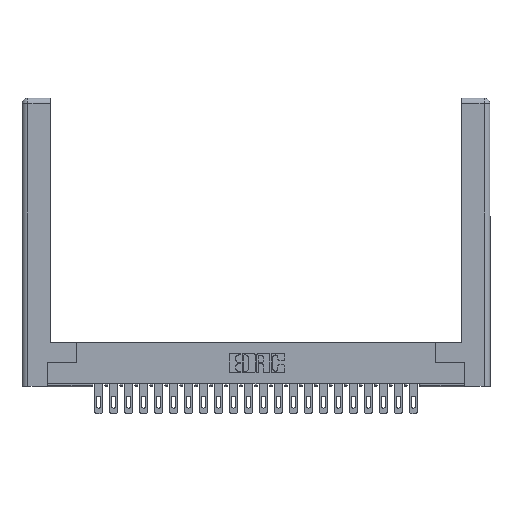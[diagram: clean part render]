
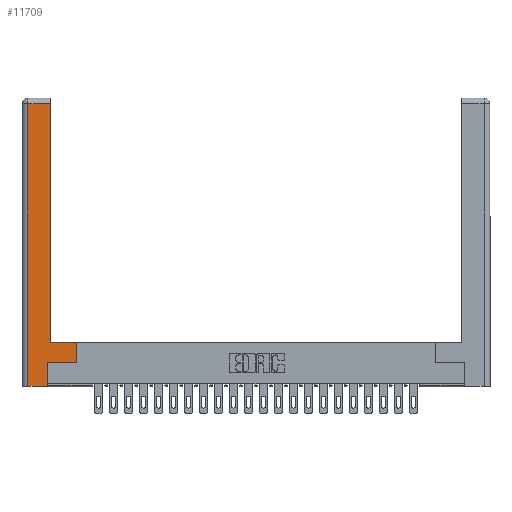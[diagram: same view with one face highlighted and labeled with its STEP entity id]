
A CAD part, top view. The second image highlights one B-rep face of the part: STEP entity #11709.
In plain terms, the highlighted planar face has unit normal (0, 0, 1).
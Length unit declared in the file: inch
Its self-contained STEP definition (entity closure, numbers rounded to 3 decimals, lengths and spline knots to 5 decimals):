
#30 = VECTOR ( 'NONE', #4873, 39.37008 ) ;
#86 = EDGE_CURVE ( 'NONE', #2580, #2665, #5890, .T. ) ;
#1006 = CARTESIAN_POINT ( 'NONE',  ( 0.0615, 2.94, 0. ) ) ;
#1077 = EDGE_CURVE ( 'NONE', #2665, #10648, #22975, .T. ) ;
#1743 = ORIENTED_EDGE ( 'NONE', *, *, #7577, .T. ) ;
#2580 = VERTEX_POINT ( 'NONE', #10593 ) ;
#2665 = VERTEX_POINT ( 'NONE', #12175 ) ;
#3704 = EDGE_LOOP ( 'NONE', ( #20453, #13679, #1743, #4742, #23100, #13297, #11654, #8114 ) ) ;
#4268 = VERTEX_POINT ( 'NONE', #21868 ) ;
#4742 = ORIENTED_EDGE ( 'NONE', *, *, #86, .T. ) ;
#4873 = DIRECTION ( 'NONE',  ( 0., 1., 0. ) ) ;
#4985 = LINE ( 'NONE', #13018, #13797 ) ;
#5576 = CARTESIAN_POINT ( 'NONE',  ( 0.565, 0.245, 0. ) ) ;
#5744 = CARTESIAN_POINT ( 'NONE',  ( 0.265, 0., 0. ) ) ;
#5890 = LINE ( 'NONE', #5744, #17512 ) ;
#6529 = DIRECTION ( 'NONE',  ( 0., 1., 0. ) ) ;
#7114 = DIRECTION ( 'NONE',  ( -1., 0., 0. ) ) ;
#7507 = VERTEX_POINT ( 'NONE', #16440 ) ;
#7577 = EDGE_CURVE ( 'NONE', #19471, #2580, #22825, .T. ) ;
#7915 = DIRECTION ( 'NONE',  ( 0., 0., -1. ) ) ;
#8114 = ORIENTED_EDGE ( 'NONE', *, *, #12169, .T. ) ;
#8278 = VECTOR ( 'NONE', #24922, 39.37008 ) ;
#8797 = EDGE_CURVE ( 'NONE', #4268, #19471, #19155, .T. ) ;
#9209 = CARTESIAN_POINT ( 'NONE',  ( 0.0615, 2.94, 0. ) ) ;
#9589 = CARTESIAN_POINT ( 'NONE',  ( 0.295, 0.45, 0. ) ) ;
#9928 = LINE ( 'NONE', #16227, #25656 ) ;
#9991 = VERTEX_POINT ( 'NONE', #5576 ) ;
#10003 = CARTESIAN_POINT ( 'NONE',  ( 0.265, 0.245, 0. ) ) ;
#10066 = AXIS2_PLACEMENT_3D ( 'NONE', #21660, #7915, #23891 ) ;
#10488 = CARTESIAN_POINT ( 'NONE',  ( 0.565, 0.45, 0. ) ) ;
#10593 = CARTESIAN_POINT ( 'NONE',  ( 0.0615, 0., 0. ) ) ;
#10648 = VERTEX_POINT ( 'NONE', #10003 ) ;
#11654 = ORIENTED_EDGE ( 'NONE', *, *, #23310, .T. ) ;
#11709 = ADVANCED_FACE ( 'NONE', ( #17361 ), #17755, .F. ) ;
#12169 = EDGE_CURVE ( 'NONE', #21334, #7507, #21245, .T. ) ;
#12175 = CARTESIAN_POINT ( 'NONE',  ( 0.265, 0., 0. ) ) ;
#13018 = CARTESIAN_POINT ( 'NONE',  ( 0.295, 3., 0. ) ) ;
#13297 = ORIENTED_EDGE ( 'NONE', *, *, #24865, .T. ) ;
#13560 = EDGE_CURVE ( 'NONE', #7507, #4268, #4985, .T. ) ;
#13679 = ORIENTED_EDGE ( 'NONE', *, *, #8797, .T. ) ;
#13797 = VECTOR ( 'NONE', #20851, 39.37008 ) ;
#16227 = CARTESIAN_POINT ( 'NONE',  ( 0.565, 0.245, 0. ) ) ;
#16386 = LINE ( 'NONE', #10488, #22650 ) ;
#16440 = CARTESIAN_POINT ( 'NONE',  ( 0.295, 0.45, 0. ) ) ;
#17361 = FACE_OUTER_BOUND ( 'NONE', #3704, .T. ) ;
#17438 = VECTOR ( 'NONE', #17587, 39.37008 ) ;
#17512 = VECTOR ( 'NONE', #17822, 39.37008 ) ;
#17587 = DIRECTION ( 'NONE',  ( -1., 0., 0. ) ) ;
#17755 = PLANE ( 'NONE',  #10066 ) ;
#17822 = DIRECTION ( 'NONE',  ( 1., 0., 0. ) ) ;
#18903 = CARTESIAN_POINT ( 'NONE',  ( 0.0615, 0., 0. ) ) ;
#19155 = LINE ( 'NONE', #9209, #20884 ) ;
#19471 = VERTEX_POINT ( 'NONE', #1006 ) ;
#20453 = ORIENTED_EDGE ( 'NONE', *, *, #13560, .T. ) ;
#20851 = DIRECTION ( 'NONE',  ( 0., 1., 0. ) ) ;
#20883 = CARTESIAN_POINT ( 'NONE',  ( 0.265, 0.245, 0. ) ) ;
#20884 = VECTOR ( 'NONE', #7114, 39.37008 ) ;
#21245 = LINE ( 'NONE', #9589, #17438 ) ;
#21334 = VERTEX_POINT ( 'NONE', #22334 ) ;
#21660 = CARTESIAN_POINT ( 'NONE',  ( 0., 0., 0. ) ) ;
#21868 = CARTESIAN_POINT ( 'NONE',  ( 0.295, 2.94, 0. ) ) ;
#22334 = CARTESIAN_POINT ( 'NONE',  ( 0.565, 0.45, 0. ) ) ;
#22650 = VECTOR ( 'NONE', #6529, 39.37008 ) ;
#22825 = LINE ( 'NONE', #18903, #8278 ) ;
#22975 = LINE ( 'NONE', #20883, #30 ) ;
#23100 = ORIENTED_EDGE ( 'NONE', *, *, #1077, .T. ) ;
#23310 = EDGE_CURVE ( 'NONE', #9991, #21334, #16386, .T. ) ;
#23891 = DIRECTION ( 'NONE',  ( -1., 0., 0. ) ) ;
#23951 = DIRECTION ( 'NONE',  ( 1., 0., 0. ) ) ;
#24865 = EDGE_CURVE ( 'NONE', #10648, #9991, #9928, .T. ) ;
#24922 = DIRECTION ( 'NONE',  ( 0., -1., 0. ) ) ;
#25656 = VECTOR ( 'NONE', #23951, 39.37008 ) ;
